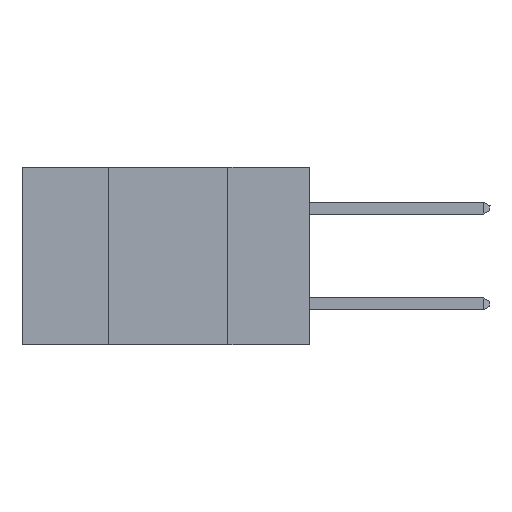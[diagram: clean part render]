
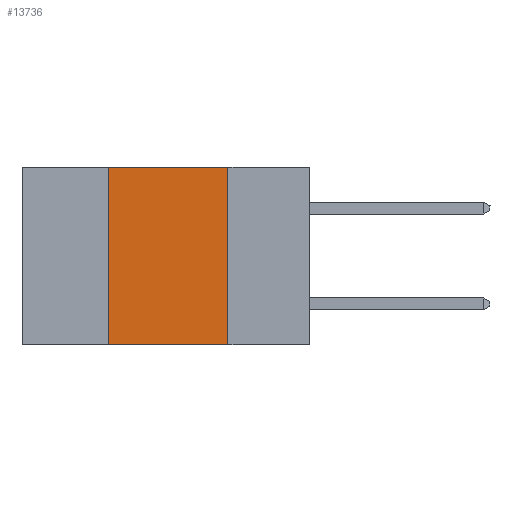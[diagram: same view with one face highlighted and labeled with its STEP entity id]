
A CAD part, left-side view. The second image highlights one B-rep face of the part: STEP entity #13736.
In plain terms, the highlighted planar face has unit normal (-1, 0, 0).
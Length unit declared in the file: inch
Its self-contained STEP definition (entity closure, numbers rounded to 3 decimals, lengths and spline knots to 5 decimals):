
#564 = ORIENTED_EDGE ( 'NONE', *, *, #2900, .F. ) ;
#933 = ORIENTED_EDGE ( 'NONE', *, *, #1143, .T. ) ;
#1077 = CARTESIAN_POINT ( 'NONE',  ( 0., 0.17, 0. ) ) ;
#1143 = EDGE_CURVE ( 'NONE', #10467, #3661, #8609, .T. ) ;
#1696 = LINE ( 'NONE', #13063, #10549 ) ;
#1715 = VECTOR ( 'NONE', #4493, 39.37008 ) ;
#1790 = EDGE_LOOP ( 'NONE', ( #8884, #564, #11980, #933 ) ) ;
#1865 = VECTOR ( 'NONE', #5266, 39.37008 ) ;
#1969 = DIRECTION ( 'NONE',  ( 0., 0., -1. ) ) ;
#2900 = EDGE_CURVE ( 'NONE', #11907, #2984, #1696, .T. ) ;
#2984 = VERTEX_POINT ( 'NONE', #9423 ) ;
#3661 = VERTEX_POINT ( 'NONE', #9029 ) ;
#4104 = CARTESIAN_POINT ( 'NONE',  ( 0., 0.42, 0. ) ) ;
#4493 = DIRECTION ( 'NONE',  ( 0., 0., -1. ) ) ;
#5266 = DIRECTION ( 'NONE',  ( 0., 0., 1. ) ) ;
#6536 = PLANE ( 'NONE',  #14067 ) ;
#6569 = EDGE_CURVE ( 'NONE', #2984, #3661, #10572, .T. ) ;
#7097 = DIRECTION ( 'NONE',  ( 0., -1., 0. ) ) ;
#7298 = CARTESIAN_POINT ( 'NONE',  ( 0., 0.6, -0.37 ) ) ;
#7407 = FACE_OUTER_BOUND ( 'NONE', #1790, .T. ) ;
#7550 = CARTESIAN_POINT ( 'NONE',  ( 0., 0.42, 0. ) ) ;
#7604 = EDGE_CURVE ( 'NONE', #10467, #11907, #11030, .T. ) ;
#7637 = CARTESIAN_POINT ( 'NONE',  ( 0., 0.6, 0. ) ) ;
#8609 = LINE ( 'NONE', #7298, #13509 ) ;
#8698 = DIRECTION ( 'NONE',  ( 1., 0., 0. ) ) ;
#8884 = ORIENTED_EDGE ( 'NONE', *, *, #6569, .F. ) ;
#9029 = CARTESIAN_POINT ( 'NONE',  ( 0., 0.17, -0.37 ) ) ;
#9423 = CARTESIAN_POINT ( 'NONE',  ( 0., 0.17, 0. ) ) ;
#10467 = VERTEX_POINT ( 'NONE', #13371 ) ;
#10549 = VECTOR ( 'NONE', #10758, 39.37008 ) ;
#10572 = LINE ( 'NONE', #1077, #1715 ) ;
#10758 = DIRECTION ( 'NONE',  ( 0., -1., 0. ) ) ;
#11030 = LINE ( 'NONE', #4104, #1865 ) ;
#11907 = VERTEX_POINT ( 'NONE', #7550 ) ;
#11980 = ORIENTED_EDGE ( 'NONE', *, *, #7604, .F. ) ;
#13063 = CARTESIAN_POINT ( 'NONE',  ( 0., 0.6, 0. ) ) ;
#13371 = CARTESIAN_POINT ( 'NONE',  ( 0., 0.42, -0.37 ) ) ;
#13509 = VECTOR ( 'NONE', #7097, 39.37008 ) ;
#13736 = ADVANCED_FACE ( 'NONE', ( #7407 ), #6536, .F. ) ;
#14067 = AXIS2_PLACEMENT_3D ( 'NONE', #7637, #8698, #1969 ) ;
